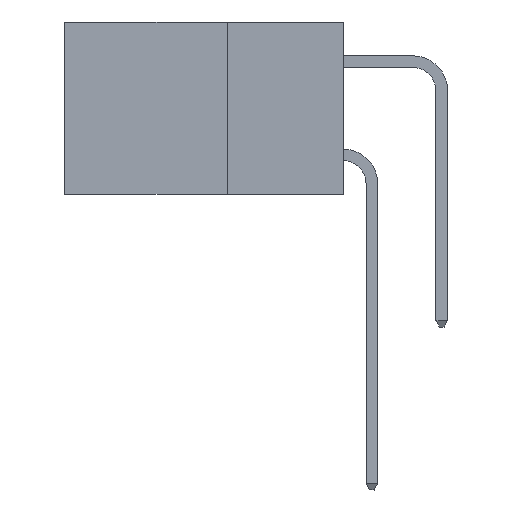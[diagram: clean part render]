
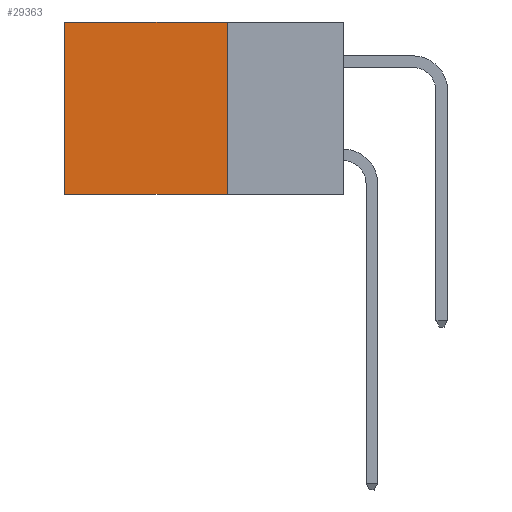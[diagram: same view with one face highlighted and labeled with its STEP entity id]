
A CAD part, left-side view. The second image highlights one B-rep face of the part: STEP entity #29363.
In plain terms, the highlighted planar face has unit normal (-1, 0, 0).
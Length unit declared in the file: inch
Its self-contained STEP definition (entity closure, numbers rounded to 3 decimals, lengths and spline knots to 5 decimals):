
#614 = CARTESIAN_POINT ( 'NONE',  ( 0.298, 0.6, 0. ) ) ;
#1416 = ORIENTED_EDGE ( 'NONE', *, *, #6310, .F. ) ;
#1464 = DIRECTION ( 'NONE',  ( 0., 0., -1. ) ) ;
#2162 = CARTESIAN_POINT ( 'NONE',  ( 0.298, 0.25, 0. ) ) ;
#2930 = DIRECTION ( 'NONE',  ( 0., 1., 0. ) ) ;
#4296 = CARTESIAN_POINT ( 'NONE',  ( 0.298, 0.6, -0.37 ) ) ;
#4959 = ORIENTED_EDGE ( 'NONE', *, *, #17669, .T. ) ;
#6310 = EDGE_CURVE ( 'NONE', #20146, #17387, #24103, .T. ) ;
#6973 = DIRECTION ( 'NONE',  ( 0., 1., 0. ) ) ;
#7270 = CARTESIAN_POINT ( 'NONE',  ( 0.298, 0.6, 0. ) ) ;
#8435 = AXIS2_PLACEMENT_3D ( 'NONE', #29701, #15761, #1464 ) ;
#9663 = DIRECTION ( 'NONE',  ( 0., 0., -1. ) ) ;
#12526 = VECTOR ( 'NONE', #9663, 39.37008 ) ;
#13304 = ORIENTED_EDGE ( 'NONE', *, *, #29369, .F. ) ;
#14365 = VERTEX_POINT ( 'NONE', #2162 ) ;
#15700 = FACE_OUTER_BOUND ( 'NONE', #17100, .T. ) ;
#15761 = DIRECTION ( 'NONE',  ( 1., 0., 0. ) ) ;
#17100 = EDGE_LOOP ( 'NONE', ( #27242, #1416, #13304, #4959 ) ) ;
#17387 = VERTEX_POINT ( 'NONE', #4296 ) ;
#17669 = EDGE_CURVE ( 'NONE', #14365, #18359, #20509, .T. ) ;
#17938 = VECTOR ( 'NONE', #6973, 39.37008 ) ;
#18359 = VERTEX_POINT ( 'NONE', #614 ) ;
#19790 = VECTOR ( 'NONE', #2930, 39.37008 ) ;
#20146 = VERTEX_POINT ( 'NONE', #28142 ) ;
#20416 = PLANE ( 'NONE',  #8435 ) ;
#20509 = LINE ( 'NONE', #21953, #19790 ) ;
#21953 = CARTESIAN_POINT ( 'NONE',  ( 0.298, 0.25, 0. ) ) ;
#22063 = CARTESIAN_POINT ( 'NONE',  ( 0.298, 0.25, -0.37 ) ) ;
#24103 = LINE ( 'NONE', #22063, #17938 ) ;
#25019 = LINE ( 'NONE', #7270, #12526 ) ;
#25161 = DIRECTION ( 'NONE',  ( 0., 0., -1. ) ) ;
#26654 = EDGE_CURVE ( 'NONE', #18359, #17387, #25019, .T. ) ;
#27242 = ORIENTED_EDGE ( 'NONE', *, *, #26654, .T. ) ;
#27381 = VECTOR ( 'NONE', #25161, 39.37008 ) ;
#27386 = CARTESIAN_POINT ( 'NONE',  ( 0.298, 0.25, 0. ) ) ;
#28142 = CARTESIAN_POINT ( 'NONE',  ( 0.298, 0.25, -0.37 ) ) ;
#28816 = LINE ( 'NONE', #27386, #27381 ) ;
#29363 = ADVANCED_FACE ( 'NONE', ( #15700 ), #20416, .F. ) ;
#29369 = EDGE_CURVE ( 'NONE', #14365, #20146, #28816, .T. ) ;
#29701 = CARTESIAN_POINT ( 'NONE',  ( 0.298, 0.25, 0. ) ) ;
